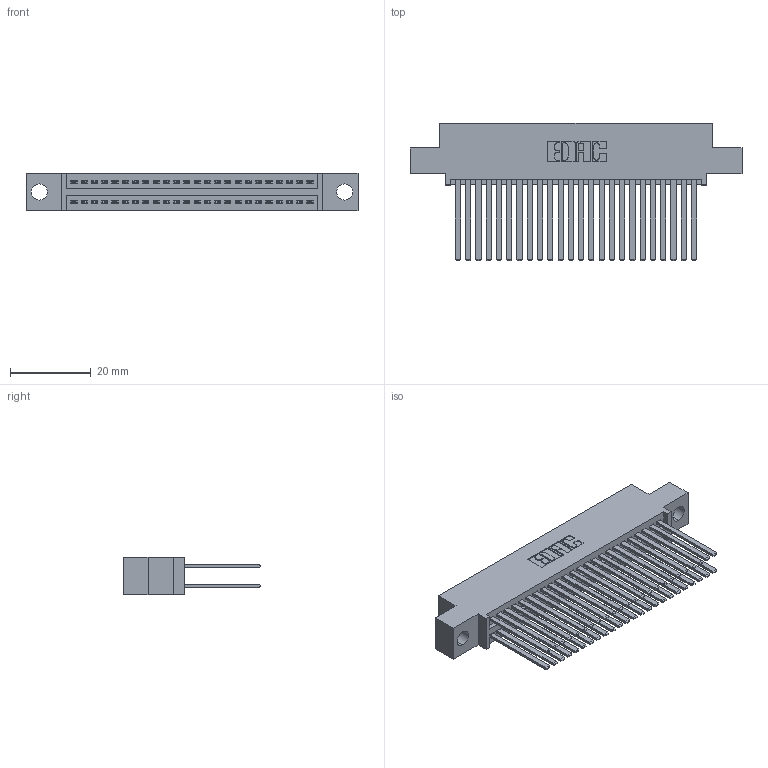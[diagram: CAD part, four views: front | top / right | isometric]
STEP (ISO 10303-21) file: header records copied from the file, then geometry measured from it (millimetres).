
FILE_DESCRIPTION (( 'STEP AP203' ), '1' );
FILE_NAME ('345-048-544-504.STEP', '2021-05-20T02:52:36', ( '' ), ( '' ), 'SwSTEP 2.0', 'SolidWorks 2020', '' );
FILE_SCHEMA (( 'CONFIG_CONTROL_DESIGN' ));
Length unit declared in the file: inch
Products named in the file (3): 345 Part_0.110 Offset - 0.156 Dia-TI; 345-048-544-504; 345-292-001_345-293-144
Assembly tree (49 placements, depth 2):
  345-048-544-504
    345 Part_0.110 Offset - 0.156 Dia-TI
    345-292-001_345-293-144  x48
Bounding box: 82.17 x 33.96 x 9.4 mm (x, y, z)
Volume: 8308.5 mm3; surface area: 13849.2 mm2
Topology: 49 solids, 49 shells, 2256 faces, 6677 edges, 4386 vertices
Faces by surface type: plane 1490, cylinder 766
Entity records: 21621 total; most frequent: CARTESIAN_POINT 3646, ORIENTED_EDGE 3578, DIRECTION 3233, EDGE_CURVE 1789, LINE 1565, VECTOR 1565, VERTEX_POINT 1190, AXIS2_PLACEMENT_3D 834
